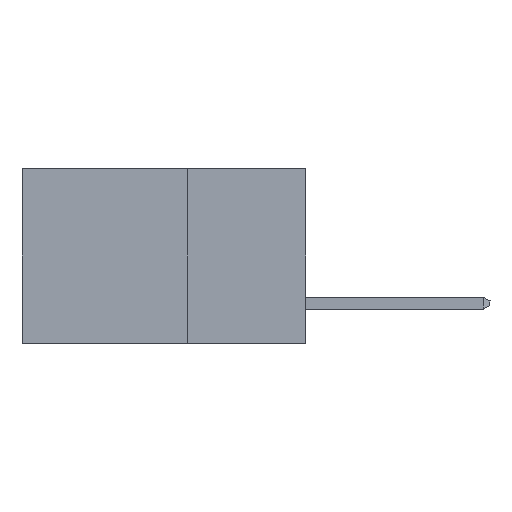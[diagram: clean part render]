
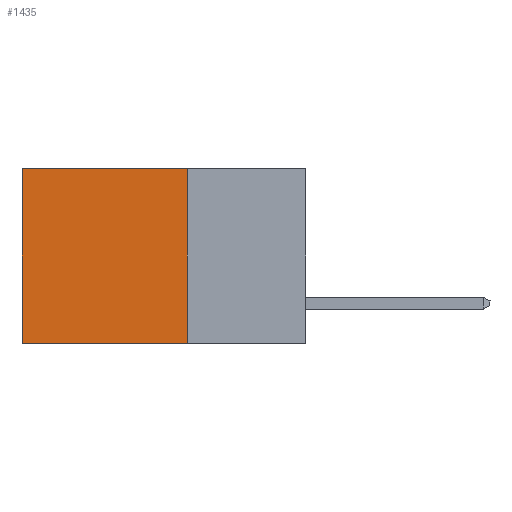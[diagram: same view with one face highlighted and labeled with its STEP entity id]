
A CAD part, left-side view. The second image highlights one B-rep face of the part: STEP entity #1435.
In plain terms, the highlighted planar face has unit normal (-1, 0, 0).
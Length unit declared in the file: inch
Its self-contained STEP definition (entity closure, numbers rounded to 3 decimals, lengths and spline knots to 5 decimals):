
#193 = LINE ( 'NONE', #11272, #12115 ) ;
#320 = CARTESIAN_POINT ( 'NONE',  ( 0.298, 0.6, 0. ) ) ;
#1435 = ADVANCED_FACE ( 'NONE', ( #18414 ), #22628, .F. ) ;
#1796 = ORIENTED_EDGE ( 'NONE', *, *, #17097, .T. ) ;
#2805 = ORIENTED_EDGE ( 'NONE', *, *, #10045, .F. ) ;
#3534 = ORIENTED_EDGE ( 'NONE', *, *, #10915, .T. ) ;
#5207 = CARTESIAN_POINT ( 'NONE',  ( 0.298, 0.25, -0.37 ) ) ;
#5245 = CARTESIAN_POINT ( 'NONE',  ( 0.298, 0.25, 0. ) ) ;
#5380 = DIRECTION ( 'NONE',  ( 0., 0., -1. ) ) ;
#5540 = DIRECTION ( 'NONE',  ( 1., 0., 0. ) ) ;
#5929 = EDGE_LOOP ( 'NONE', ( #3534, #2805, #10711, #1796 ) ) ;
#7856 = LINE ( 'NONE', #5207, #12946 ) ;
#8584 = VERTEX_POINT ( 'NONE', #11982 ) ;
#10045 = EDGE_CURVE ( 'NONE', #24963, #8584, #7856, .T. ) ;
#10464 = VERTEX_POINT ( 'NONE', #320 ) ;
#10711 = ORIENTED_EDGE ( 'NONE', *, *, #19674, .F. ) ;
#10915 = EDGE_CURVE ( 'NONE', #10464, #8584, #18291, .T. ) ;
#11272 = CARTESIAN_POINT ( 'NONE',  ( 0.298, 0.25, 0. ) ) ;
#11982 = CARTESIAN_POINT ( 'NONE',  ( 0.298, 0.6, -0.37 ) ) ;
#12053 = VECTOR ( 'NONE', #20054, 39.37008 ) ;
#12115 = VECTOR ( 'NONE', #15615, 39.37008 ) ;
#12946 = VECTOR ( 'NONE', #20428, 39.37008 ) ;
#13813 = VERTEX_POINT ( 'NONE', #5245 ) ;
#14013 = CARTESIAN_POINT ( 'NONE',  ( 0.298, 0.25, 0. ) ) ;
#15423 = AXIS2_PLACEMENT_3D ( 'NONE', #14013, #5540, #18648 ) ;
#15615 = DIRECTION ( 'NONE',  ( 0., 0., -1. ) ) ;
#15935 = VECTOR ( 'NONE', #5380, 39.37008 ) ;
#17097 = EDGE_CURVE ( 'NONE', #13813, #10464, #17448, .T. ) ;
#17448 = LINE ( 'NONE', #22224, #12053 ) ;
#18291 = LINE ( 'NONE', #24797, #15935 ) ;
#18414 = FACE_OUTER_BOUND ( 'NONE', #5929, .T. ) ;
#18648 = DIRECTION ( 'NONE',  ( 0., 0., -1. ) ) ;
#19674 = EDGE_CURVE ( 'NONE', #13813, #24963, #193, .T. ) ;
#20054 = DIRECTION ( 'NONE',  ( 0., 1., 0. ) ) ;
#20428 = DIRECTION ( 'NONE',  ( 0., 1., 0. ) ) ;
#22224 = CARTESIAN_POINT ( 'NONE',  ( 0.298, 0.25, 0. ) ) ;
#22628 = PLANE ( 'NONE',  #15423 ) ;
#24355 = CARTESIAN_POINT ( 'NONE',  ( 0.298, 0.25, -0.37 ) ) ;
#24797 = CARTESIAN_POINT ( 'NONE',  ( 0.298, 0.6, 0. ) ) ;
#24963 = VERTEX_POINT ( 'NONE', #24355 ) ;
